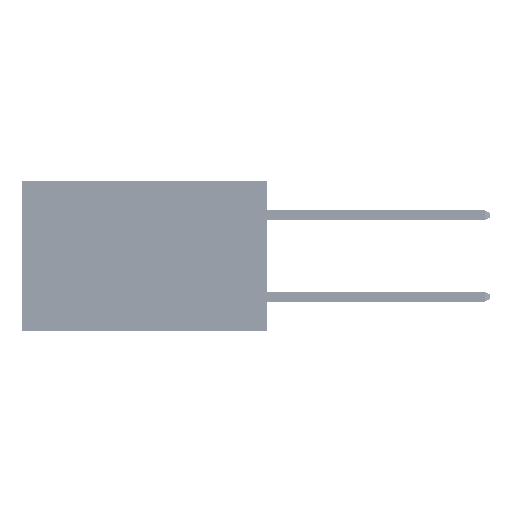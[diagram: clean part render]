
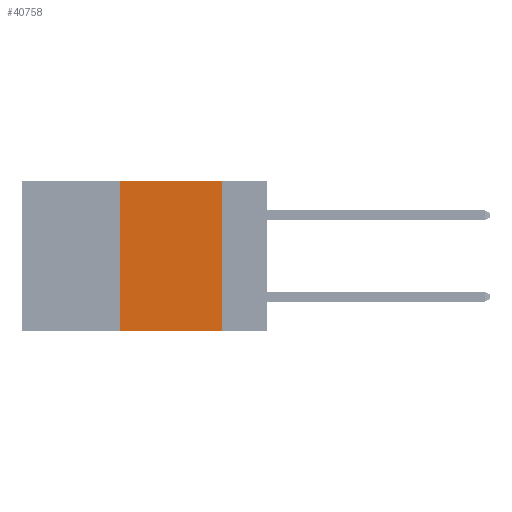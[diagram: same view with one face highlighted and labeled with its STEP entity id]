
A CAD part, left-side view. The second image highlights one B-rep face of the part: STEP entity #40758.
In plain terms, the highlighted planar face has unit normal (-1, 0, 0).
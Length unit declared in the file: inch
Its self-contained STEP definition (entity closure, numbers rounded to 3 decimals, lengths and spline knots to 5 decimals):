
#3101 = EDGE_CURVE ( 'NONE', #28709, #19875, #34253, .T. ) ;
#7082 = CARTESIAN_POINT ( 'NONE',  ( 0., 0.36, -0.37 ) ) ;
#8955 = DIRECTION ( 'NONE',  ( 0., 0., 1. ) ) ;
#9373 = FACE_OUTER_BOUND ( 'NONE', #25070, .T. ) ;
#9849 = ORIENTED_EDGE ( 'NONE', *, *, #3101, .T. ) ;
#10703 = CARTESIAN_POINT ( 'NONE',  ( 0., 0.6, 0. ) ) ;
#11518 = VECTOR ( 'NONE', #8955, 39.37008 ) ;
#12479 = CARTESIAN_POINT ( 'NONE',  ( 0., 0.6, -0.37 ) ) ;
#13148 = LINE ( 'NONE', #21367, #30086 ) ;
#14206 = DIRECTION ( 'NONE',  ( 0., 0., -1. ) ) ;
#14363 = CARTESIAN_POINT ( 'NONE',  ( 0., 0.11, 0. ) ) ;
#14971 = VECTOR ( 'NONE', #38849, 39.37008 ) ;
#15152 = DIRECTION ( 'NONE',  ( 1., 0., 0. ) ) ;
#18159 = AXIS2_PLACEMENT_3D ( 'NONE', #38905, #15152, #14206 ) ;
#19875 = VERTEX_POINT ( 'NONE', #27970 ) ;
#20090 = CARTESIAN_POINT ( 'NONE',  ( 0., 0.36, 0. ) ) ;
#21367 = CARTESIAN_POINT ( 'NONE',  ( 0., 0.11, 0. ) ) ;
#23158 = EDGE_CURVE ( 'NONE', #24287, #29787, #43217, .T. ) ;
#24144 = PLANE ( 'NONE',  #18159 ) ;
#24287 = VERTEX_POINT ( 'NONE', #46131 ) ;
#24847 = ORIENTED_EDGE ( 'NONE', *, *, #23158, .F. ) ;
#25070 = EDGE_LOOP ( 'NONE', ( #39317, #24847, #30249, #9849 ) ) ;
#26759 = DIRECTION ( 'NONE',  ( 0., -1., 0. ) ) ;
#27970 = CARTESIAN_POINT ( 'NONE',  ( 0., 0.11, -0.37 ) ) ;
#28709 = VERTEX_POINT ( 'NONE', #7082 ) ;
#29787 = VERTEX_POINT ( 'NONE', #14363 ) ;
#30086 = VECTOR ( 'NONE', #47274, 39.37008 ) ;
#30249 = ORIENTED_EDGE ( 'NONE', *, *, #31148, .F. ) ;
#31148 = EDGE_CURVE ( 'NONE', #28709, #24287, #42121, .T. ) ;
#32065 = EDGE_CURVE ( 'NONE', #29787, #19875, #13148, .T. ) ;
#34253 = LINE ( 'NONE', #12479, #43714 ) ;
#38849 = DIRECTION ( 'NONE',  ( 0., -1., 0. ) ) ;
#38905 = CARTESIAN_POINT ( 'NONE',  ( 0., 0.6, 0. ) ) ;
#39317 = ORIENTED_EDGE ( 'NONE', *, *, #32065, .F. ) ;
#40758 = ADVANCED_FACE ( 'NONE', ( #9373 ), #24144, .F. ) ;
#42121 = LINE ( 'NONE', #20090, #11518 ) ;
#43217 = LINE ( 'NONE', #10703, #14971 ) ;
#43714 = VECTOR ( 'NONE', #26759, 39.37008 ) ;
#46131 = CARTESIAN_POINT ( 'NONE',  ( 0., 0.36, 0. ) ) ;
#47274 = DIRECTION ( 'NONE',  ( 0., 0., -1. ) ) ;
